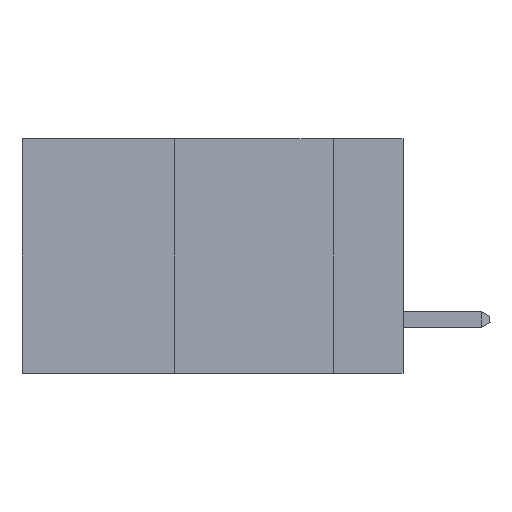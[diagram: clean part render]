
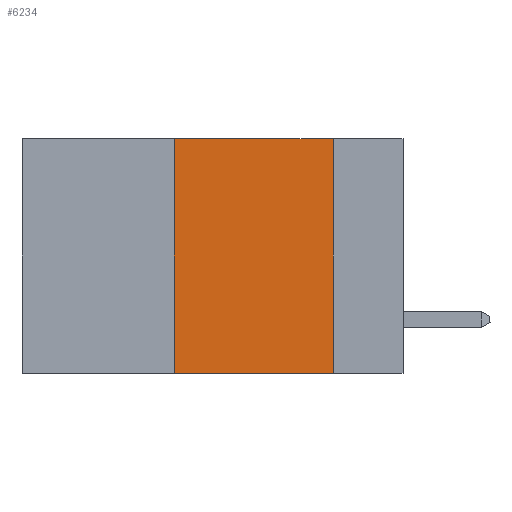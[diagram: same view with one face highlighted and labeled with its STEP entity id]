
A CAD part, left-side view. The second image highlights one B-rep face of the part: STEP entity #6234.
In plain terms, the highlighted planar face has unit normal (-1, 0, 0).
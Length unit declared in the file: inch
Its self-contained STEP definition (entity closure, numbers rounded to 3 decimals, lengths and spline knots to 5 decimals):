
#52 = LINE ( 'NONE', #10150, #548 ) ;
#548 = VECTOR ( 'NONE', #2685, 39.37008 ) ;
#745 = VERTEX_POINT ( 'NONE', #2095 ) ;
#1003 = ORIENTED_EDGE ( 'NONE', *, *, #17265, .F. ) ;
#1403 = DIRECTION ( 'NONE',  ( 0., 0., -1. ) ) ;
#1407 = EDGE_LOOP ( 'NONE', ( #3789, #1003, #13488, #7217 ) ) ;
#2095 = CARTESIAN_POINT ( 'NONE',  ( 0., 0.11, 0. ) ) ;
#2507 = LINE ( 'NONE', #14149, #9991 ) ;
#2685 = DIRECTION ( 'NONE',  ( 0., -1., 0. ) ) ;
#3108 = EDGE_CURVE ( 'NONE', #19092, #8327, #12658, .T. ) ;
#3150 = AXIS2_PLACEMENT_3D ( 'NONE', #16660, #10338, #1403 ) ;
#3789 = ORIENTED_EDGE ( 'NONE', *, *, #16279, .F. ) ;
#5025 = VERTEX_POINT ( 'NONE', #18200 ) ;
#6234 = ADVANCED_FACE ( 'NONE', ( #16078 ), #15150, .F. ) ;
#6381 = DIRECTION ( 'NONE',  ( 0., 0., -1. ) ) ;
#7217 = ORIENTED_EDGE ( 'NONE', *, *, #3108, .T. ) ;
#8327 = VERTEX_POINT ( 'NONE', #18348 ) ;
#8778 = VECTOR ( 'NONE', #6381, 39.37008 ) ;
#8919 = EDGE_CURVE ( 'NONE', #19092, #5025, #2507, .T. ) ;
#9383 = CARTESIAN_POINT ( 'NONE',  ( 0., 0.36, -0.37 ) ) ;
#9991 = VECTOR ( 'NONE', #15710, 39.37008 ) ;
#10150 = CARTESIAN_POINT ( 'NONE',  ( 0., 0.6, 0. ) ) ;
#10338 = DIRECTION ( 'NONE',  ( 1., 0., 0. ) ) ;
#11400 = CARTESIAN_POINT ( 'NONE',  ( 0., 0.6, -0.37 ) ) ;
#12658 = LINE ( 'NONE', #11400, #14311 ) ;
#13465 = LINE ( 'NONE', #13823, #8778 ) ;
#13488 = ORIENTED_EDGE ( 'NONE', *, *, #8919, .F. ) ;
#13823 = CARTESIAN_POINT ( 'NONE',  ( 0., 0.11, 0. ) ) ;
#14149 = CARTESIAN_POINT ( 'NONE',  ( 0., 0.36, 0. ) ) ;
#14311 = VECTOR ( 'NONE', #14740, 39.37008 ) ;
#14740 = DIRECTION ( 'NONE',  ( 0., -1., 0. ) ) ;
#15150 = PLANE ( 'NONE',  #3150 ) ;
#15710 = DIRECTION ( 'NONE',  ( 0., 0., 1. ) ) ;
#16078 = FACE_OUTER_BOUND ( 'NONE', #1407, .T. ) ;
#16279 = EDGE_CURVE ( 'NONE', #745, #8327, #13465, .T. ) ;
#16660 = CARTESIAN_POINT ( 'NONE',  ( 0., 0.6, 0. ) ) ;
#17265 = EDGE_CURVE ( 'NONE', #5025, #745, #52, .T. ) ;
#18200 = CARTESIAN_POINT ( 'NONE',  ( 0., 0.36, 0. ) ) ;
#18348 = CARTESIAN_POINT ( 'NONE',  ( 0., 0.11, -0.37 ) ) ;
#19092 = VERTEX_POINT ( 'NONE', #9383 ) ;
